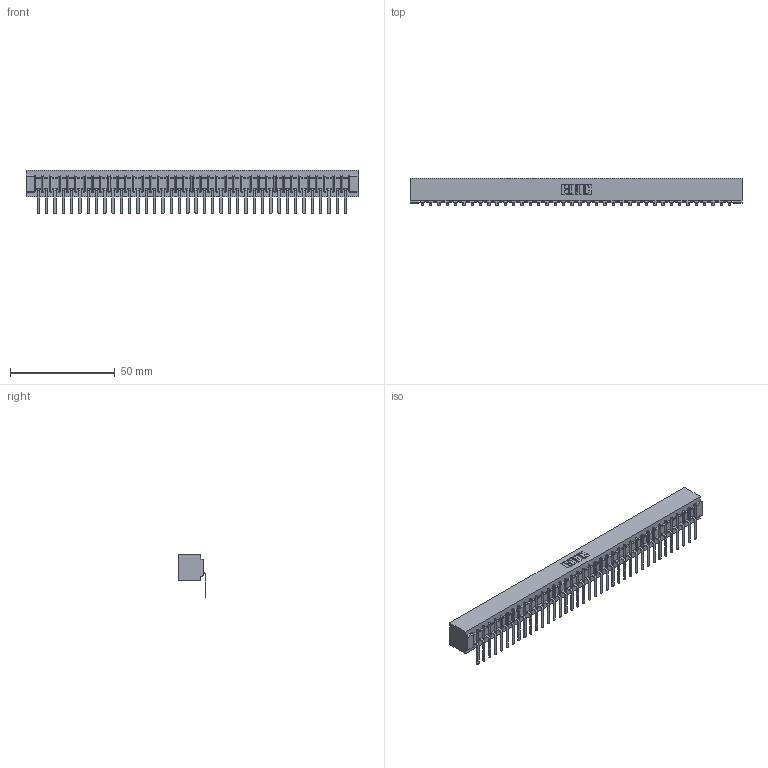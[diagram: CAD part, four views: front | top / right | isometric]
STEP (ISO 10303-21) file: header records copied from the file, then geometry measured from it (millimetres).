
FILE_DESCRIPTION (( 'STEP AP203' ), '1' );
FILE_NAME ('357-038-557-101.STEP', '2019-09-17T08:04:14', ( '' ), ( '' ), 'SwSTEP 2.0', 'SolidWorks 2016', '' );
FILE_SCHEMA (( 'CONFIG_CONTROL_DESIGN' ));
Length unit declared in the file: inch
Products named in the file (3): 307-290-002_557; 357-038-557-101; 307 Part_No Mounting Lugs
Assembly tree (39 placements, depth 2):
  357-038-557-101
    307 Part_No Mounting Lugs
    307-290-002_557  x38
Bounding box: 158.45 x 13.32 x 20.66 mm (x, y, z)
Volume: 17586.1 mm3; surface area: 23040.6 mm2
Topology: 39 solids, 39 shells, 3113 faces, 9571 edges, 6274 vertices
Faces by surface type: plane 1852, cylinder 1183, sphere 78
Entity records: 33646 total; most frequent: CARTESIAN_POINT 5676, ORIENTED_EDGE 5666, DIRECTION 5515, EDGE_CURVE 2833, VECTOR 2169, LINE 2169, VERTEX_POINT 1834, AXIS2_PLACEMENT_3D 1673
